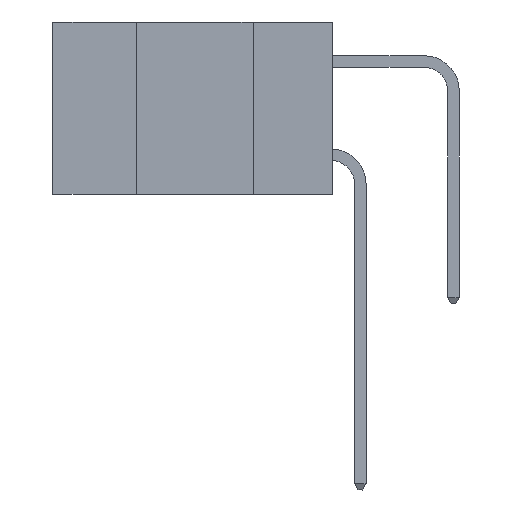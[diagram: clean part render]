
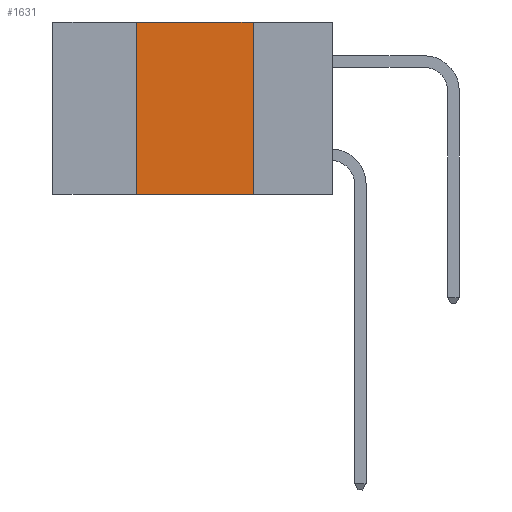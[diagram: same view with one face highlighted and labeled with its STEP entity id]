
A CAD part, left-side view. The second image highlights one B-rep face of the part: STEP entity #1631.
In plain terms, the highlighted planar face has unit normal (-1, 0, 0).
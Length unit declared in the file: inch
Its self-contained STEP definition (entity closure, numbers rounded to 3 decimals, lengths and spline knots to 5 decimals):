
#232 = VECTOR ( 'NONE', #5421, 39.37008 ) ;
#912 = VERTEX_POINT ( 'NONE', #3468 ) ;
#1214 = EDGE_CURVE ( 'NONE', #4118, #9558, #11694, .T. ) ;
#1631 = ADVANCED_FACE ( 'NONE', ( #6183 ), #11539, .F. ) ;
#2995 = VECTOR ( 'NONE', #3750, 39.37008 ) ;
#3468 = CARTESIAN_POINT ( 'NONE',  ( 0., 0.17, -0.37 ) ) ;
#3479 = AXIS2_PLACEMENT_3D ( 'NONE', #10240, #10201, #5648 ) ;
#3750 = DIRECTION ( 'NONE',  ( 0., 0., 1. ) ) ;
#4118 = VERTEX_POINT ( 'NONE', #8279 ) ;
#4316 = VERTEX_POINT ( 'NONE', #5883 ) ;
#4476 = CARTESIAN_POINT ( 'NONE',  ( 0., 0.6, -0.37 ) ) ;
#5359 = CARTESIAN_POINT ( 'NONE',  ( 0., 0.17, 0. ) ) ;
#5421 = DIRECTION ( 'NONE',  ( 0., -1., 0. ) ) ;
#5648 = DIRECTION ( 'NONE',  ( 0., 0., -1. ) ) ;
#5883 = CARTESIAN_POINT ( 'NONE',  ( 0., 0.42, -0.37 ) ) ;
#6183 = FACE_OUTER_BOUND ( 'NONE', #10189, .T. ) ;
#6500 = VECTOR ( 'NONE', #10644, 39.37008 ) ;
#6560 = ORIENTED_EDGE ( 'NONE', *, *, #10527, .F. ) ;
#6658 = CARTESIAN_POINT ( 'NONE',  ( 0., 0.42, 0. ) ) ;
#6878 = ORIENTED_EDGE ( 'NONE', *, *, #11932, .F. ) ;
#6964 = CARTESIAN_POINT ( 'NONE',  ( 0., 0.17, 0. ) ) ;
#7544 = LINE ( 'NONE', #5359, #12086 ) ;
#8255 = LINE ( 'NONE', #4476, #232 ) ;
#8279 = CARTESIAN_POINT ( 'NONE',  ( 0., 0.42, 0. ) ) ;
#9558 = VERTEX_POINT ( 'NONE', #6964 ) ;
#10189 = EDGE_LOOP ( 'NONE', ( #6560, #11480, #6878, #11750 ) ) ;
#10201 = DIRECTION ( 'NONE',  ( 1., 0., 0. ) ) ;
#10240 = CARTESIAN_POINT ( 'NONE',  ( 0., 0.6, 0. ) ) ;
#10527 = EDGE_CURVE ( 'NONE', #9558, #912, #7544, .T. ) ;
#10544 = LINE ( 'NONE', #6658, #2995 ) ;
#10644 = DIRECTION ( 'NONE',  ( 0., -1., 0. ) ) ;
#10671 = EDGE_CURVE ( 'NONE', #4316, #912, #8255, .T. ) ;
#11164 = CARTESIAN_POINT ( 'NONE',  ( 0., 0.6, 0. ) ) ;
#11480 = ORIENTED_EDGE ( 'NONE', *, *, #1214, .F. ) ;
#11539 = PLANE ( 'NONE',  #3479 ) ;
#11694 = LINE ( 'NONE', #11164, #6500 ) ;
#11750 = ORIENTED_EDGE ( 'NONE', *, *, #10671, .T. ) ;
#11826 = DIRECTION ( 'NONE',  ( 0., 0., -1. ) ) ;
#11932 = EDGE_CURVE ( 'NONE', #4316, #4118, #10544, .T. ) ;
#12086 = VECTOR ( 'NONE', #11826, 39.37008 ) ;
